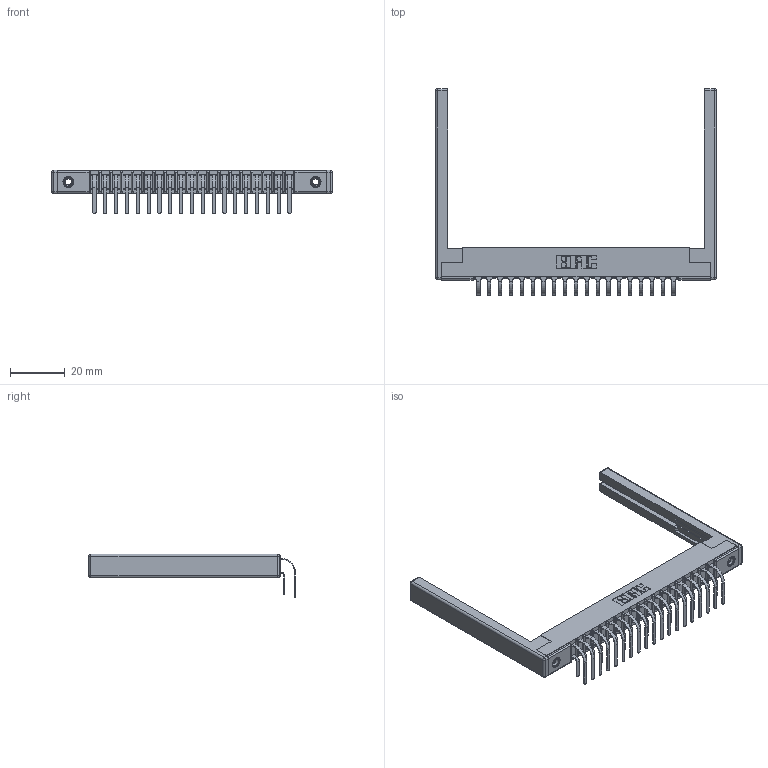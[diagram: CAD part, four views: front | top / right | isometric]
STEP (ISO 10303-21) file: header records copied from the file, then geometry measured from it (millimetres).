
FILE_DESCRIPTION (( 'STEP AP203' ), '1' );
FILE_NAME ('307-038-459-268.STEP', '2022-07-07T16:41:35', ( '' ), ( '' ), 'SwSTEP 2.0', 'SolidWorks 2020', '' );
FILE_SCHEMA (( 'CONFIG_CONTROL_DESIGN' ));
Length unit declared in the file: inch
Products named in the file (6): 307-290-001_559 - 2 (Single); 307 Part_.156 Dia Mounting Holes; 307-220-068; 307-038-459-268; 345-250-001_345-250-001-102; 307-290-001_558 559 - 1 (Single)
Assembly tree (43 placements, depth 2):
  307-038-459-268
    307 Part_.156 Dia Mounting Holes
    307-290-001_558 559 - 1 (Single)  x19
    307-290-001_559 - 2 (Single)  x19
    307-220-068  x2
    345-250-001_345-250-001-102  x2
Bounding box: 102.72 x 75.48 x 16.08 mm (x, y, z)
Volume: 11423.6 mm3; surface area: 16802.6 mm2
Topology: 43 solids, 43 shells, 2192 faces, 6109 edges, 3946 vertices
Faces by surface type: plane 1412, cylinder 716, sphere 48, cone 12, torus 4
Entity records: 23938 total; most frequent: CARTESIAN_POINT 3902, ORIENTED_EDGE 3856, DIRECTION 3846, EDGE_CURVE 1928, LINE 1466, VECTOR 1466, VERTEX_POINT 1246, AXIS2_PLACEMENT_3D 1190
